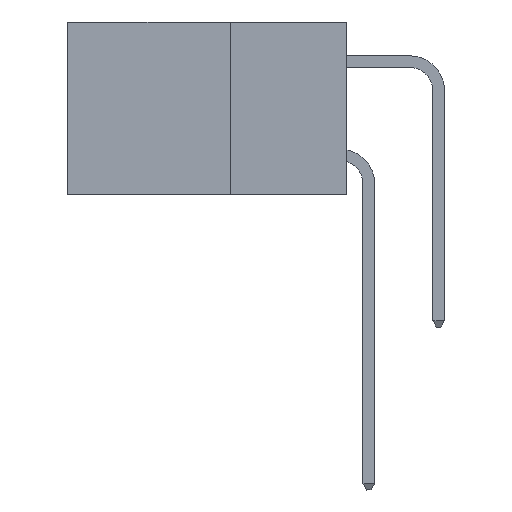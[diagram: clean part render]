
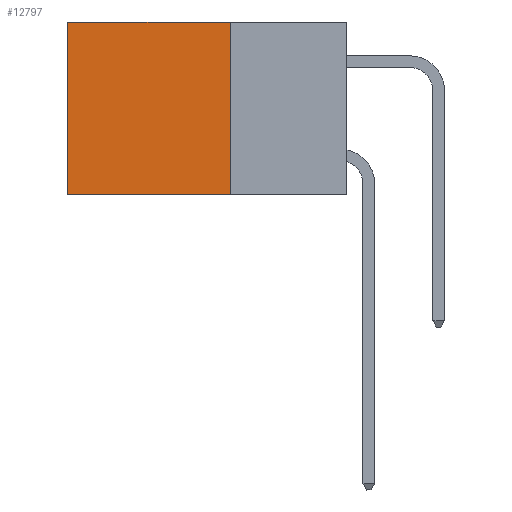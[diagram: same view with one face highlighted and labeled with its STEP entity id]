
A CAD part, left-side view. The second image highlights one B-rep face of the part: STEP entity #12797.
In plain terms, the highlighted planar face has unit normal (-1, 0, 0).
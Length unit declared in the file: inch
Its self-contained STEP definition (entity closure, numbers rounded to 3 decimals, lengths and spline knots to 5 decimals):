
#78 = DIRECTION ( 'NONE',  ( 1., 0., 0. ) ) ;
#1113 = VERTEX_POINT ( 'NONE', #16507 ) ;
#1257 = LINE ( 'NONE', #11451, #5231 ) ;
#1706 = CARTESIAN_POINT ( 'NONE',  ( 0.2875, 0.25, 0. ) ) ;
#1984 = VERTEX_POINT ( 'NONE', #12563 ) ;
#2732 = DIRECTION ( 'NONE',  ( 0., 0., -1. ) ) ;
#2978 = EDGE_LOOP ( 'NONE', ( #4511, #14615, #12970, #16352 ) ) ;
#3960 = FACE_OUTER_BOUND ( 'NONE', #2978, .T. ) ;
#4354 = DIRECTION ( 'NONE',  ( 0., 0., -1. ) ) ;
#4498 = AXIS2_PLACEMENT_3D ( 'NONE', #5906, #78, #8643 ) ;
#4511 = ORIENTED_EDGE ( 'NONE', *, *, #17792, .T. ) ;
#5231 = VECTOR ( 'NONE', #12884, 39.37008 ) ;
#5365 = VERTEX_POINT ( 'NONE', #1706 ) ;
#5906 = CARTESIAN_POINT ( 'NONE',  ( 0.2875, 0.25, 0. ) ) ;
#5949 = LINE ( 'NONE', #16527, #18146 ) ;
#8522 = CARTESIAN_POINT ( 'NONE',  ( 0.2875, 0.6, 0. ) ) ;
#8643 = DIRECTION ( 'NONE',  ( 0., 0., -1. ) ) ;
#8670 = VERTEX_POINT ( 'NONE', #8522 ) ;
#9415 = VECTOR ( 'NONE', #2732, 39.37008 ) ;
#9589 = EDGE_CURVE ( 'NONE', #5365, #8670, #1257, .T. ) ;
#9861 = LINE ( 'NONE', #18092, #9415 ) ;
#10419 = LINE ( 'NONE', #11308, #17569 ) ;
#11308 = CARTESIAN_POINT ( 'NONE',  ( 0.2875, 0.25, 0. ) ) ;
#11451 = CARTESIAN_POINT ( 'NONE',  ( 0.2875, 0.25, 0. ) ) ;
#11602 = EDGE_CURVE ( 'NONE', #5365, #1984, #10419, .T. ) ;
#12563 = CARTESIAN_POINT ( 'NONE',  ( 0.2875, 0.25, -0.37 ) ) ;
#12797 = ADVANCED_FACE ( 'NONE', ( #3960 ), #13024, .F. ) ;
#12884 = DIRECTION ( 'NONE',  ( 0., 1., 0. ) ) ;
#12970 = ORIENTED_EDGE ( 'NONE', *, *, #11602, .F. ) ;
#13024 = PLANE ( 'NONE',  #4498 ) ;
#13789 = DIRECTION ( 'NONE',  ( 0., 1., 0. ) ) ;
#14615 = ORIENTED_EDGE ( 'NONE', *, *, #16513, .F. ) ;
#16352 = ORIENTED_EDGE ( 'NONE', *, *, #9589, .T. ) ;
#16507 = CARTESIAN_POINT ( 'NONE',  ( 0.2875, 0.6, -0.37 ) ) ;
#16513 = EDGE_CURVE ( 'NONE', #1984, #1113, #5949, .T. ) ;
#16527 = CARTESIAN_POINT ( 'NONE',  ( 0.2875, 0.25, -0.37 ) ) ;
#17569 = VECTOR ( 'NONE', #4354, 39.37008 ) ;
#17792 = EDGE_CURVE ( 'NONE', #8670, #1113, #9861, .T. ) ;
#18092 = CARTESIAN_POINT ( 'NONE',  ( 0.2875, 0.6, 0. ) ) ;
#18146 = VECTOR ( 'NONE', #13789, 39.37008 ) ;
